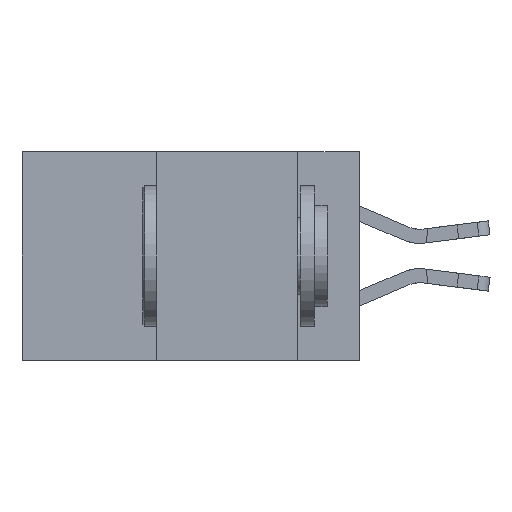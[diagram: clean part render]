
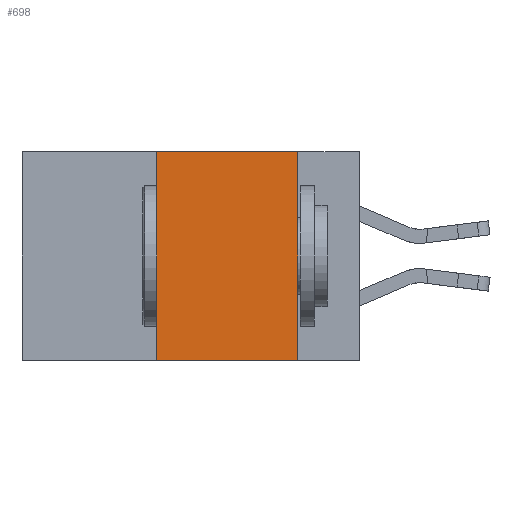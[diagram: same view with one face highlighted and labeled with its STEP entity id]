
A CAD part, left-side view. The second image highlights one B-rep face of the part: STEP entity #698.
In plain terms, the highlighted planar face has unit normal (-1, 0, 0).
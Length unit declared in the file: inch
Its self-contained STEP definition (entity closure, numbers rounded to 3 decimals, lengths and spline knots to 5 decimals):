
#297 = VECTOR ( 'NONE', #14868, 39.37008 ) ;
#470 = ORIENTED_EDGE ( 'NONE', *, *, #18297, .F. ) ;
#672 = VECTOR ( 'NONE', #16468, 39.37008 ) ;
#698 = ADVANCED_FACE ( 'NONE', ( #9748 ), #3473, .F. ) ;
#1193 = LINE ( 'NONE', #13270, #672 ) ;
#1720 = DIRECTION ( 'NONE',  ( 0., 0., -1. ) ) ;
#1732 = DIRECTION ( 'NONE',  ( 0., 0., 1. ) ) ;
#3473 = PLANE ( 'NONE',  #19191 ) ;
#3698 = VERTEX_POINT ( 'NONE', #12002 ) ;
#3960 = VECTOR ( 'NONE', #5243, 39.37008 ) ;
#4810 = VECTOR ( 'NONE', #1732, 39.37008 ) ;
#5000 = ORIENTED_EDGE ( 'NONE', *, *, #18869, .T. ) ;
#5119 = DIRECTION ( 'NONE',  ( 1., 0., 0. ) ) ;
#5171 = CARTESIAN_POINT ( 'NONE',  ( 0., 0.11, 0. ) ) ;
#5243 = DIRECTION ( 'NONE',  ( 0., 0., -1. ) ) ;
#5718 = EDGE_LOOP ( 'NONE', ( #7501, #13582, #470, #5000 ) ) ;
#5819 = CARTESIAN_POINT ( 'NONE',  ( 0., 0.11, -0.37 ) ) ;
#6362 = VERTEX_POINT ( 'NONE', #15304 ) ;
#7266 = EDGE_CURVE ( 'NONE', #3698, #12824, #16408, .T. ) ;
#7501 = ORIENTED_EDGE ( 'NONE', *, *, #7266, .F. ) ;
#8311 = CARTESIAN_POINT ( 'NONE',  ( 0., 0.6, 0. ) ) ;
#9529 = CARTESIAN_POINT ( 'NONE',  ( 0., 0.36, -0.37 ) ) ;
#9748 = FACE_OUTER_BOUND ( 'NONE', #5718, .T. ) ;
#9853 = VERTEX_POINT ( 'NONE', #9529 ) ;
#10573 = LINE ( 'NONE', #11760, #297 ) ;
#11760 = CARTESIAN_POINT ( 'NONE',  ( 0., 0.6, 0. ) ) ;
#12002 = CARTESIAN_POINT ( 'NONE',  ( 0., 0.11, 0. ) ) ;
#12824 = VERTEX_POINT ( 'NONE', #5819 ) ;
#13270 = CARTESIAN_POINT ( 'NONE',  ( 0., 0.6, -0.37 ) ) ;
#13582 = ORIENTED_EDGE ( 'NONE', *, *, #20982, .F. ) ;
#14868 = DIRECTION ( 'NONE',  ( 0., -1., 0. ) ) ;
#15304 = CARTESIAN_POINT ( 'NONE',  ( 0., 0.36, 0. ) ) ;
#16408 = LINE ( 'NONE', #5171, #3960 ) ;
#16468 = DIRECTION ( 'NONE',  ( 0., -1., 0. ) ) ;
#17514 = LINE ( 'NONE', #19704, #4810 ) ;
#18297 = EDGE_CURVE ( 'NONE', #9853, #6362, #17514, .T. ) ;
#18869 = EDGE_CURVE ( 'NONE', #9853, #12824, #1193, .T. ) ;
#19191 = AXIS2_PLACEMENT_3D ( 'NONE', #8311, #5119, #1720 ) ;
#19704 = CARTESIAN_POINT ( 'NONE',  ( 0., 0.36, 0. ) ) ;
#20982 = EDGE_CURVE ( 'NONE', #6362, #3698, #10573, .T. ) ;
